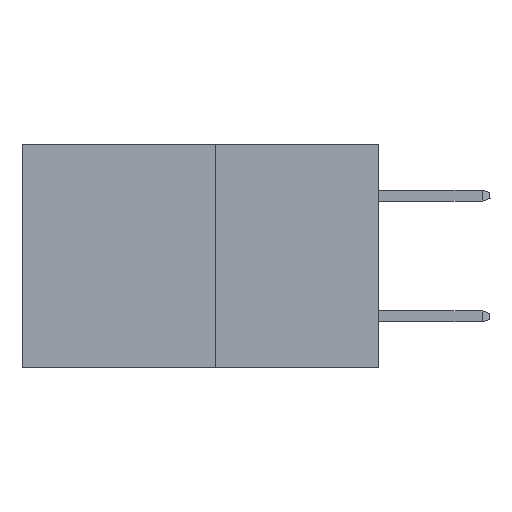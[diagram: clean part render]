
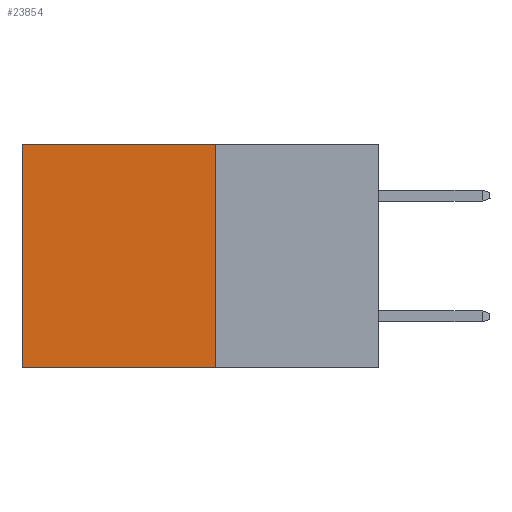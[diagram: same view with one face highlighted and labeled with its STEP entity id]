
A CAD part, left-side view. The second image highlights one B-rep face of the part: STEP entity #23854.
In plain terms, the highlighted planar face has unit normal (-1, 0, 0).
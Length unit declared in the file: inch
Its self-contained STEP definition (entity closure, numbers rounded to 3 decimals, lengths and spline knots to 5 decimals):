
#510 = DIRECTION ( 'NONE',  ( 0., 0., -1. ) ) ;
#630 = ORIENTED_EDGE ( 'NONE', *, *, #6468, .F. ) ;
#754 = VECTOR ( 'NONE', #755, 39.37008 ) ;
#755 = DIRECTION ( 'NONE',  ( 0., 1., 0. ) ) ;
#956 = CARTESIAN_POINT ( 'NONE',  ( 0.277, 0.59, 0. ) ) ;
#2165 = CARTESIAN_POINT ( 'NONE',  ( 0.277, 0.27, -0.37 ) ) ;
#2290 = ORIENTED_EDGE ( 'NONE', *, *, #18565, .T. ) ;
#4852 = VERTEX_POINT ( 'NONE', #22895 ) ;
#5581 = ORIENTED_EDGE ( 'NONE', *, *, #30414, .T. ) ;
#6038 = FACE_OUTER_BOUND ( 'NONE', #21541, .T. ) ;
#6468 = EDGE_CURVE ( 'NONE', #28099, #4852, #18843, .T. ) ;
#9000 = VERTEX_POINT ( 'NONE', #13005 ) ;
#9478 = DIRECTION ( 'NONE',  ( 0., 0., -1. ) ) ;
#11058 = DIRECTION ( 'NONE',  ( 0., 0., -1. ) ) ;
#12564 = VECTOR ( 'NONE', #9478, 39.37008 ) ;
#12613 = CARTESIAN_POINT ( 'NONE',  ( 0.277, 0.27, -0.37 ) ) ;
#13005 = CARTESIAN_POINT ( 'NONE',  ( 0.277, 0.59, -0.37 ) ) ;
#13613 = LINE ( 'NONE', #24613, #754 ) ;
#13775 = VECTOR ( 'NONE', #25186, 39.37008 ) ;
#14993 = DIRECTION ( 'NONE',  ( 1., 0., 0. ) ) ;
#17026 = VERTEX_POINT ( 'NONE', #956 ) ;
#17902 = CARTESIAN_POINT ( 'NONE',  ( 0.277, 0.27, 0. ) ) ;
#18485 = AXIS2_PLACEMENT_3D ( 'NONE', #12613, #14993, #510 ) ;
#18565 = EDGE_CURVE ( 'NONE', #17026, #9000, #25240, .T. ) ;
#18843 = LINE ( 'NONE', #2165, #12564 ) ;
#18967 = VECTOR ( 'NONE', #11058, 39.37008 ) ;
#19829 = ORIENTED_EDGE ( 'NONE', *, *, #28709, .F. ) ;
#21541 = EDGE_LOOP ( 'NONE', ( #2290, #19829, #630, #5581 ) ) ;
#22777 = CARTESIAN_POINT ( 'NONE',  ( 0.277, 0.27, -0.37 ) ) ;
#22895 = CARTESIAN_POINT ( 'NONE',  ( 0.277, 0.27, -0.37 ) ) ;
#23854 = ADVANCED_FACE ( 'NONE', ( #6038 ), #26731, .F. ) ;
#24613 = CARTESIAN_POINT ( 'NONE',  ( 0.277, 0.27, 0. ) ) ;
#25186 = DIRECTION ( 'NONE',  ( 0., 1., 0. ) ) ;
#25216 = CARTESIAN_POINT ( 'NONE',  ( 0.277, 0.59, -0.37 ) ) ;
#25240 = LINE ( 'NONE', #25216, #18967 ) ;
#26319 = LINE ( 'NONE', #22777, #13775 ) ;
#26731 = PLANE ( 'NONE',  #18485 ) ;
#28099 = VERTEX_POINT ( 'NONE', #17902 ) ;
#28709 = EDGE_CURVE ( 'NONE', #4852, #9000, #26319, .T. ) ;
#30414 = EDGE_CURVE ( 'NONE', #28099, #17026, #13613, .T. ) ;
